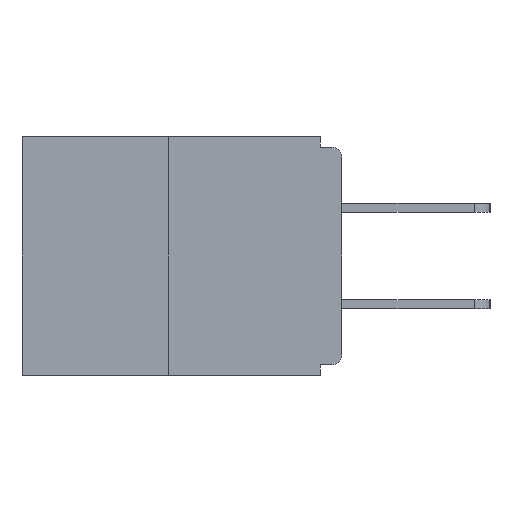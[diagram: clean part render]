
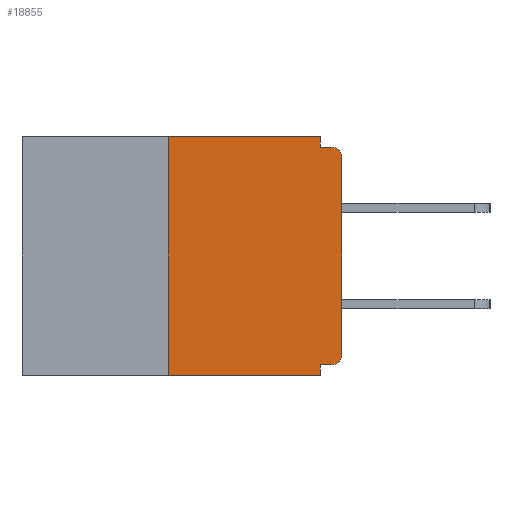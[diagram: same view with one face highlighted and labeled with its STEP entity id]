
A CAD part, left-side view. The second image highlights one B-rep face of the part: STEP entity #18855.
In plain terms, the highlighted planar face has unit normal (-1, 0, 0).
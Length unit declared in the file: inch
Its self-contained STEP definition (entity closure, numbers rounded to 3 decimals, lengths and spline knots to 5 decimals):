
#1005 = VECTOR ( 'NONE', #8847, 39.37008 ) ;
#1045 = DIRECTION ( 'NONE',  ( 0., 1., 0. ) ) ;
#1151 = VERTEX_POINT ( 'NONE', #5300 ) ;
#1175 = CARTESIAN_POINT ( 'NONE',  ( 0., 0.46, 0. ) ) ;
#1358 = DIRECTION ( 'NONE',  ( -1., 0., 0. ) ) ;
#1743 = VERTEX_POINT ( 'NONE', #14623 ) ;
#1914 = EDGE_CURVE ( 'NONE', #8815, #17896, #17065, .T. ) ;
#2052 = DIRECTION ( 'NONE',  ( -1., 0., 0. ) ) ;
#2563 = LINE ( 'NONE', #18585, #12215 ) ;
#2589 = VERTEX_POINT ( 'NONE', #14901 ) ;
#2737 = EDGE_CURVE ( 'NONE', #1151, #5025, #16778, .T. ) ;
#3081 = FACE_OUTER_BOUND ( 'NONE', #7323, .T. ) ;
#4010 = CARTESIAN_POINT ( 'NONE',  ( 0., 0.25, 0. ) ) ;
#4028 = EDGE_CURVE ( 'NONE', #5787, #2589, #16396, .T. ) ;
#4073 = DIRECTION ( 'NONE',  ( 0., -1., 0. ) ) ;
#4215 = CARTESIAN_POINT ( 'NONE',  ( 0., 0., -0.313 ) ) ;
#4876 = VECTOR ( 'NONE', #1045, 39.37008 ) ;
#5024 = CARTESIAN_POINT ( 'NONE',  ( 0., 0.015, -0.015 ) ) ;
#5025 = VERTEX_POINT ( 'NONE', #9525 ) ;
#5127 = EDGE_CURVE ( 'NONE', #10316, #5025, #2563, .T. ) ;
#5231 = VECTOR ( 'NONE', #11480, 39.37008 ) ;
#5300 = CARTESIAN_POINT ( 'NONE',  ( 0., 0.25, -0.343 ) ) ;
#5357 = ORIENTED_EDGE ( 'NONE', *, *, #10769, .F. ) ;
#5412 = CARTESIAN_POINT ( 'NONE',  ( 0., 0.25, 0. ) ) ;
#5424 = DIRECTION ( 'NONE',  ( 0., 0., 1. ) ) ;
#5787 = VERTEX_POINT ( 'NONE', #4215 ) ;
#6028 = DIRECTION ( 'NONE',  ( 0., -1., 0. ) ) ;
#6267 = AXIS2_PLACEMENT_3D ( 'NONE', #9272, #2052, #15172 ) ;
#6319 = EDGE_CURVE ( 'NONE', #1151, #8815, #11024, .T. ) ;
#6727 = ORIENTED_EDGE ( 'NONE', *, *, #5127, .F. ) ;
#6834 = CARTESIAN_POINT ( 'NONE',  ( 0., 0.015, -0.328 ) ) ;
#7323 = EDGE_LOOP ( 'NONE', ( #9744, #18810, #9422, #6727, #9345, #17014, #13502, #11105, #5357, #14987 ) ) ;
#7502 = CARTESIAN_POINT ( 'NONE',  ( 0., 0.031, -0.328 ) ) ;
#8724 = VERTEX_POINT ( 'NONE', #6834 ) ;
#8813 = LINE ( 'NONE', #18768, #4876 ) ;
#8815 = VERTEX_POINT ( 'NONE', #5412 ) ;
#8847 = DIRECTION ( 'NONE',  ( 0., -1., 0. ) ) ;
#9272 = CARTESIAN_POINT ( 'NONE',  ( 0., 0.015, -0.03 ) ) ;
#9345 = ORIENTED_EDGE ( 'NONE', *, *, #9808, .F. ) ;
#9422 = ORIENTED_EDGE ( 'NONE', *, *, #2737, .T. ) ;
#9525 = CARTESIAN_POINT ( 'NONE',  ( 0., 0.031, -0.343 ) ) ;
#9744 = ORIENTED_EDGE ( 'NONE', *, *, #1914, .F. ) ;
#9808 = EDGE_CURVE ( 'NONE', #8724, #10316, #8813, .T. ) ;
#9942 = CARTESIAN_POINT ( 'NONE',  ( 0., 0.46, -0.343 ) ) ;
#9954 = PLANE ( 'NONE',  #11515 ) ;
#10316 = VERTEX_POINT ( 'NONE', #7502 ) ;
#10390 = LINE ( 'NONE', #18805, #1005 ) ;
#10467 = VECTOR ( 'NONE', #16040, 39.37008 ) ;
#10759 = LINE ( 'NONE', #17224, #5231 ) ;
#10769 = EDGE_CURVE ( 'NONE', #1743, #18453, #10390, .T. ) ;
#11024 = LINE ( 'NONE', #4010, #18512 ) ;
#11105 = ORIENTED_EDGE ( 'NONE', *, *, #16234, .T. ) ;
#11480 = DIRECTION ( 'NONE',  ( 0., 0., -1. ) ) ;
#11515 = AXIS2_PLACEMENT_3D ( 'NONE', #1175, #15914, #17128 ) ;
#12215 = VECTOR ( 'NONE', #18459, 39.37008 ) ;
#12590 = AXIS2_PLACEMENT_3D ( 'NONE', #12829, #1358, #12772 ) ;
#12772 = DIRECTION ( 'NONE',  ( 0., 0., -1. ) ) ;
#12829 = CARTESIAN_POINT ( 'NONE',  ( 0., 0.015, -0.313 ) ) ;
#13212 = VECTOR ( 'NONE', #6028, 39.37008 ) ;
#13394 = VECTOR ( 'NONE', #4073, 39.37008 ) ;
#13502 = ORIENTED_EDGE ( 'NONE', *, *, #4028, .T. ) ;
#14623 = CARTESIAN_POINT ( 'NONE',  ( 0., 0.031, -0.015 ) ) ;
#14625 = CIRCLE ( 'NONE', #6267, 0.015 ) ;
#14680 = CARTESIAN_POINT ( 'NONE',  ( 0., 0.46, 0. ) ) ;
#14783 = CIRCLE ( 'NONE', #12590, 0.015 ) ;
#14901 = CARTESIAN_POINT ( 'NONE',  ( 0., 0., -0.03 ) ) ;
#14987 = ORIENTED_EDGE ( 'NONE', *, *, #16940, .F. ) ;
#15172 = DIRECTION ( 'NONE',  ( 0., 0., -1. ) ) ;
#15914 = DIRECTION ( 'NONE',  ( 1., 0., 0. ) ) ;
#16040 = DIRECTION ( 'NONE',  ( 0., 0., 1. ) ) ;
#16234 = EDGE_CURVE ( 'NONE', #2589, #18453, #14625, .T. ) ;
#16396 = LINE ( 'NONE', #18838, #10467 ) ;
#16778 = LINE ( 'NONE', #9942, #13394 ) ;
#16940 = EDGE_CURVE ( 'NONE', #17896, #1743, #10759, .T. ) ;
#17014 = ORIENTED_EDGE ( 'NONE', *, *, #18871, .T. ) ;
#17065 = LINE ( 'NONE', #14680, #13212 ) ;
#17128 = DIRECTION ( 'NONE',  ( 0., 0., -1. ) ) ;
#17224 = CARTESIAN_POINT ( 'NONE',  ( 0., 0.031, 0. ) ) ;
#17820 = CARTESIAN_POINT ( 'NONE',  ( 0., 0.031, 0. ) ) ;
#17896 = VERTEX_POINT ( 'NONE', #17820 ) ;
#18453 = VERTEX_POINT ( 'NONE', #5024 ) ;
#18459 = DIRECTION ( 'NONE',  ( 0., 0., -1. ) ) ;
#18512 = VECTOR ( 'NONE', #5424, 39.37008 ) ;
#18585 = CARTESIAN_POINT ( 'NONE',  ( 0., 0.031, -0.343 ) ) ;
#18768 = CARTESIAN_POINT ( 'NONE',  ( 0., 0., -0.328 ) ) ;
#18805 = CARTESIAN_POINT ( 'NONE',  ( 0., 0., -0.015 ) ) ;
#18810 = ORIENTED_EDGE ( 'NONE', *, *, #6319, .F. ) ;
#18838 = CARTESIAN_POINT ( 'NONE',  ( 0., 0., 0. ) ) ;
#18855 = ADVANCED_FACE ( 'NONE', ( #3081 ), #9954, .F. ) ;
#18871 = EDGE_CURVE ( 'NONE', #8724, #5787, #14783, .T. ) ;
